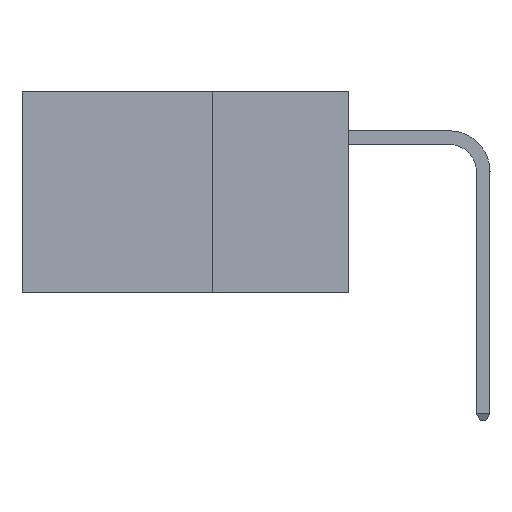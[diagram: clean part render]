
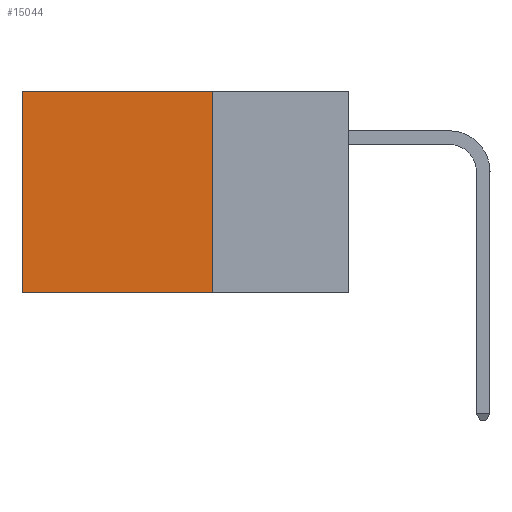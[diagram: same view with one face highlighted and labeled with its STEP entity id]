
A CAD part, left-side view. The second image highlights one B-rep face of the part: STEP entity #15044.
In plain terms, the highlighted planar face has unit normal (-1, 0, 0).
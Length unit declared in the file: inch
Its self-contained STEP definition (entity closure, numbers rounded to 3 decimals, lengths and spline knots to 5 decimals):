
#1494 = DIRECTION ( 'NONE',  ( 0., 0., -1. ) ) ;
#2475 = VECTOR ( 'NONE', #34036, 39.37008 ) ;
#3423 = CARTESIAN_POINT ( 'NONE',  ( 0.2875, 0.25, 0. ) ) ;
#3502 = EDGE_CURVE ( 'NONE', #12926, #14175, #11395, .T. ) ;
#4635 = EDGE_LOOP ( 'NONE', ( #25535, #27194, #31117, #22157 ) ) ;
#5468 = DIRECTION ( 'NONE',  ( 0., 1., 0. ) ) ;
#6122 = AXIS2_PLACEMENT_3D ( 'NONE', #24498, #15960, #36045 ) ;
#10326 = LINE ( 'NONE', #11015, #2475 ) ;
#11015 = CARTESIAN_POINT ( 'NONE',  ( 0.2875, 0.25, -0.37 ) ) ;
#11306 = EDGE_CURVE ( 'NONE', #14175, #35342, #29077, .T. ) ;
#11395 = LINE ( 'NONE', #28702, #18159 ) ;
#12926 = VERTEX_POINT ( 'NONE', #34796 ) ;
#14175 = VERTEX_POINT ( 'NONE', #31622 ) ;
#15044 = ADVANCED_FACE ( 'NONE', ( #21171 ), #18722, .F. ) ;
#15960 = DIRECTION ( 'NONE',  ( 1., 0., 0. ) ) ;
#16099 = CARTESIAN_POINT ( 'NONE',  ( 0.2875, 0.6, 0. ) ) ;
#18159 = VECTOR ( 'NONE', #5468, 39.37008 ) ;
#18722 = PLANE ( 'NONE',  #6122 ) ;
#19325 = EDGE_CURVE ( 'NONE', #29406, #35342, #10326, .T. ) ;
#21171 = FACE_OUTER_BOUND ( 'NONE', #4635, .T. ) ;
#22157 = ORIENTED_EDGE ( 'NONE', *, *, #3502, .T. ) ;
#24405 = EDGE_CURVE ( 'NONE', #12926, #29406, #33587, .T. ) ;
#24498 = CARTESIAN_POINT ( 'NONE',  ( 0.2875, 0.25, 0. ) ) ;
#25053 = VECTOR ( 'NONE', #26687, 39.37008 ) ;
#25535 = ORIENTED_EDGE ( 'NONE', *, *, #11306, .T. ) ;
#26687 = DIRECTION ( 'NONE',  ( 0., 0., -1. ) ) ;
#27053 = CARTESIAN_POINT ( 'NONE',  ( 0.2875, 0.6, -0.37 ) ) ;
#27194 = ORIENTED_EDGE ( 'NONE', *, *, #19325, .F. ) ;
#28177 = VECTOR ( 'NONE', #1494, 39.37008 ) ;
#28702 = CARTESIAN_POINT ( 'NONE',  ( 0.2875, 0.25, 0. ) ) ;
#29077 = LINE ( 'NONE', #16099, #28177 ) ;
#29406 = VERTEX_POINT ( 'NONE', #35238 ) ;
#31117 = ORIENTED_EDGE ( 'NONE', *, *, #24405, .F. ) ;
#31622 = CARTESIAN_POINT ( 'NONE',  ( 0.2875, 0.6, 0. ) ) ;
#33587 = LINE ( 'NONE', #3423, #25053 ) ;
#34036 = DIRECTION ( 'NONE',  ( 0., 1., 0. ) ) ;
#34796 = CARTESIAN_POINT ( 'NONE',  ( 0.2875, 0.25, 0. ) ) ;
#35238 = CARTESIAN_POINT ( 'NONE',  ( 0.2875, 0.25, -0.37 ) ) ;
#35342 = VERTEX_POINT ( 'NONE', #27053 ) ;
#36045 = DIRECTION ( 'NONE',  ( 0., 0., -1. ) ) ;
